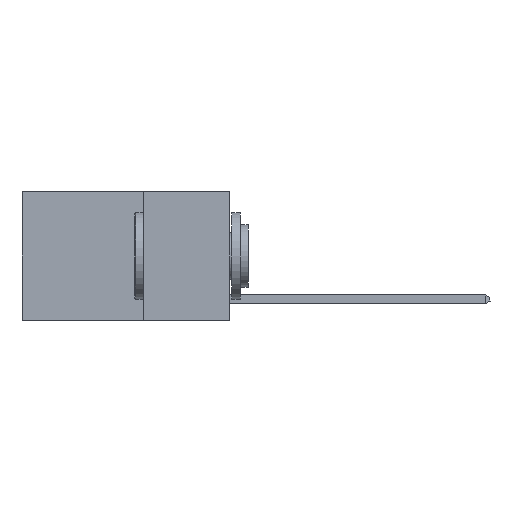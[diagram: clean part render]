
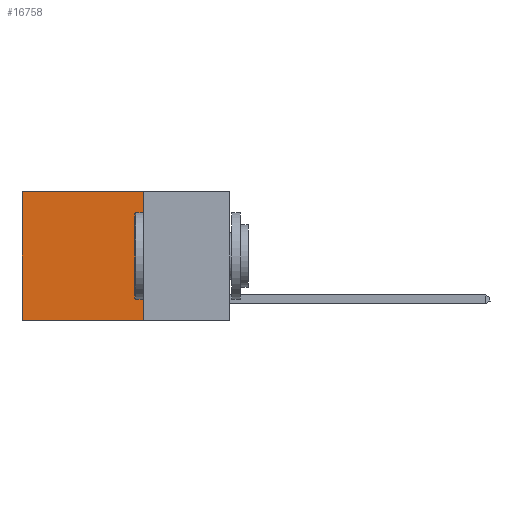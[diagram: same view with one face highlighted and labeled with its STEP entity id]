
A CAD part, left-side view. The second image highlights one B-rep face of the part: STEP entity #16758.
In plain terms, the highlighted planar face has unit normal (-1, 0, 0).
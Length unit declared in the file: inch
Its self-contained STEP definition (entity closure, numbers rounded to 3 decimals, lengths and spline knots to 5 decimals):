
#1648 = FACE_OUTER_BOUND ( 'NONE', #8207, .T. ) ;
#1806 = VERTEX_POINT ( 'NONE', #9498 ) ;
#2550 = EDGE_CURVE ( 'NONE', #1806, #15647, #6748, .T. ) ;
#4281 = DIRECTION ( 'NONE',  ( 0., 0., -1. ) ) ;
#6497 = DIRECTION ( 'NONE',  ( 1., 0., 0. ) ) ;
#6606 = VERTEX_POINT ( 'NONE', #13005 ) ;
#6748 = LINE ( 'NONE', #20703, #15650 ) ;
#7237 = CARTESIAN_POINT ( 'NONE',  ( 0.2625, 0.25, 0. ) ) ;
#7600 = EDGE_CURVE ( 'NONE', #25531, #1806, #13031, .T. ) ;
#7779 = CARTESIAN_POINT ( 'NONE',  ( 0.2625, 0.25, 0. ) ) ;
#7783 = CARTESIAN_POINT ( 'NONE',  ( 0.2625, 0.25, 0. ) ) ;
#8207 = EDGE_LOOP ( 'NONE', ( #13467, #15979, #24558, #20398 ) ) ;
#9424 = EDGE_CURVE ( 'NONE', #6606, #15647, #14335, .T. ) ;
#9498 = CARTESIAN_POINT ( 'NONE',  ( 0.2625, 0.6, 0. ) ) ;
#9904 = DIRECTION ( 'NONE',  ( 0., 0., -1. ) ) ;
#13005 = CARTESIAN_POINT ( 'NONE',  ( 0.2625, 0.25, -0.37 ) ) ;
#13031 = LINE ( 'NONE', #7237, #24252 ) ;
#13467 = ORIENTED_EDGE ( 'NONE', *, *, #2550, .T. ) ;
#13593 = DIRECTION ( 'NONE',  ( 0., 1., 0. ) ) ;
#14335 = LINE ( 'NONE', #26547, #26933 ) ;
#14512 = DIRECTION ( 'NONE',  ( 0., 0., -1. ) ) ;
#14790 = PLANE ( 'NONE',  #24139 ) ;
#15647 = VERTEX_POINT ( 'NONE', #24574 ) ;
#15650 = VECTOR ( 'NONE', #4281, 39.37008 ) ;
#15979 = ORIENTED_EDGE ( 'NONE', *, *, #9424, .F. ) ;
#16479 = VECTOR ( 'NONE', #9904, 39.37008 ) ;
#16758 = ADVANCED_FACE ( 'NONE', ( #1648 ), #14790, .F. ) ;
#16999 = DIRECTION ( 'NONE',  ( 0., 1., 0. ) ) ;
#18784 = LINE ( 'NONE', #7779, #16479 ) ;
#20398 = ORIENTED_EDGE ( 'NONE', *, *, #7600, .T. ) ;
#20703 = CARTESIAN_POINT ( 'NONE',  ( 0.2625, 0.6, 0. ) ) ;
#23117 = CARTESIAN_POINT ( 'NONE',  ( 0.2625, 0.25, 0. ) ) ;
#24139 = AXIS2_PLACEMENT_3D ( 'NONE', #23117, #6497, #14512 ) ;
#24252 = VECTOR ( 'NONE', #13593, 39.37008 ) ;
#24558 = ORIENTED_EDGE ( 'NONE', *, *, #26675, .F. ) ;
#24574 = CARTESIAN_POINT ( 'NONE',  ( 0.2625, 0.6, -0.37 ) ) ;
#25531 = VERTEX_POINT ( 'NONE', #7783 ) ;
#26547 = CARTESIAN_POINT ( 'NONE',  ( 0.2625, 0.25, -0.37 ) ) ;
#26675 = EDGE_CURVE ( 'NONE', #25531, #6606, #18784, .T. ) ;
#26933 = VECTOR ( 'NONE', #16999, 39.37008 ) ;
